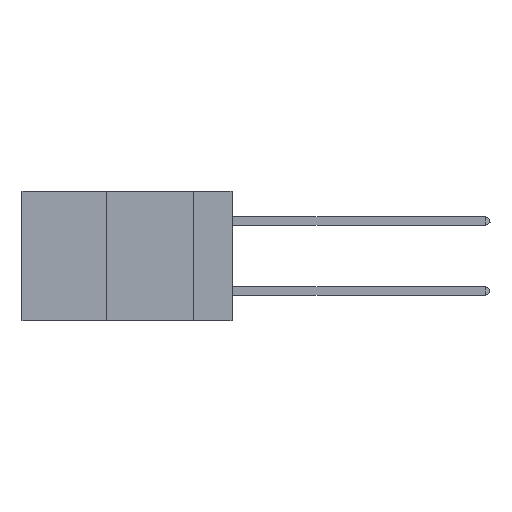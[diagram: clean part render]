
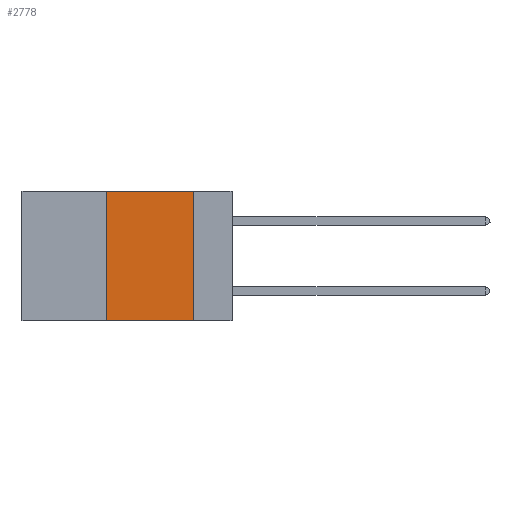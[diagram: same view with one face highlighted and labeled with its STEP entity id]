
A CAD part, left-side view. The second image highlights one B-rep face of the part: STEP entity #2778.
In plain terms, the highlighted planar face has unit normal (-1, 0, 0).
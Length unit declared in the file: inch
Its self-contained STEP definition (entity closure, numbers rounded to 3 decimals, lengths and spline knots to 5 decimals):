
#57 = ORIENTED_EDGE ( 'NONE', *, *, #5723, .T. ) ;
#198 = LINE ( 'NONE', #2515, #1228 ) ;
#922 = VERTEX_POINT ( 'NONE', #4172 ) ;
#1119 = FACE_OUTER_BOUND ( 'NONE', #1220, .T. ) ;
#1220 = EDGE_LOOP ( 'NONE', ( #2285, #11088, #4271, #57 ) ) ;
#1228 = VECTOR ( 'NONE', #1696, 39.37008 ) ;
#1696 = DIRECTION ( 'NONE',  ( 0., 0., -1. ) ) ;
#2285 = ORIENTED_EDGE ( 'NONE', *, *, #10602, .F. ) ;
#2515 = CARTESIAN_POINT ( 'NONE',  ( 0., 0.11, 0. ) ) ;
#2778 = ADVANCED_FACE ( 'NONE', ( #1119 ), #4220, .F. ) ;
#3095 = VERTEX_POINT ( 'NONE', #11785 ) ;
#3162 = DIRECTION ( 'NONE',  ( 1., 0., 0. ) ) ;
#3276 = DIRECTION ( 'NONE',  ( 0., 0., -1. ) ) ;
#3334 = VERTEX_POINT ( 'NONE', #4539 ) ;
#3736 = CARTESIAN_POINT ( 'NONE',  ( 0., 0.36, 0. ) ) ;
#4172 = CARTESIAN_POINT ( 'NONE',  ( 0., 0.36, 0. ) ) ;
#4220 = PLANE ( 'NONE',  #8983 ) ;
#4257 = VERTEX_POINT ( 'NONE', #11300 ) ;
#4271 = ORIENTED_EDGE ( 'NONE', *, *, #8057, .F. ) ;
#4539 = CARTESIAN_POINT ( 'NONE',  ( 0., 0.11, 0. ) ) ;
#5059 = CARTESIAN_POINT ( 'NONE',  ( 0., 0.6, 0. ) ) ;
#5373 = DIRECTION ( 'NONE',  ( 0., -1., 0. ) ) ;
#5626 = LINE ( 'NONE', #9967, #7661 ) ;
#5723 = EDGE_CURVE ( 'NONE', #4257, #3095, #5626, .T. ) ;
#5974 = VECTOR ( 'NONE', #9433, 39.37008 ) ;
#7102 = DIRECTION ( 'NONE',  ( 0., -1., 0. ) ) ;
#7661 = VECTOR ( 'NONE', #5373, 39.37008 ) ;
#7707 = VECTOR ( 'NONE', #7102, 39.37008 ) ;
#8057 = EDGE_CURVE ( 'NONE', #4257, #922, #9666, .T. ) ;
#8983 = AXIS2_PLACEMENT_3D ( 'NONE', #5059, #3162, #3276 ) ;
#9035 = LINE ( 'NONE', #11831, #7707 ) ;
#9433 = DIRECTION ( 'NONE',  ( 0., 0., 1. ) ) ;
#9666 = LINE ( 'NONE', #3736, #5974 ) ;
#9822 = EDGE_CURVE ( 'NONE', #922, #3334, #9035, .T. ) ;
#9967 = CARTESIAN_POINT ( 'NONE',  ( 0., 0.6, -0.37 ) ) ;
#10602 = EDGE_CURVE ( 'NONE', #3334, #3095, #198, .T. ) ;
#11088 = ORIENTED_EDGE ( 'NONE', *, *, #9822, .F. ) ;
#11300 = CARTESIAN_POINT ( 'NONE',  ( 0., 0.36, -0.37 ) ) ;
#11785 = CARTESIAN_POINT ( 'NONE',  ( 0., 0.11, -0.37 ) ) ;
#11831 = CARTESIAN_POINT ( 'NONE',  ( 0., 0.6, 0. ) ) ;
